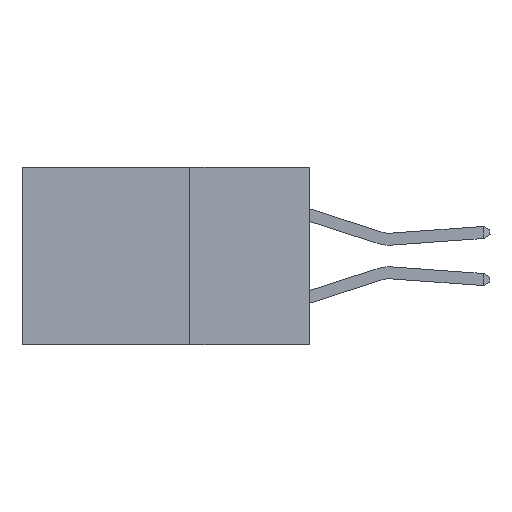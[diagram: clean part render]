
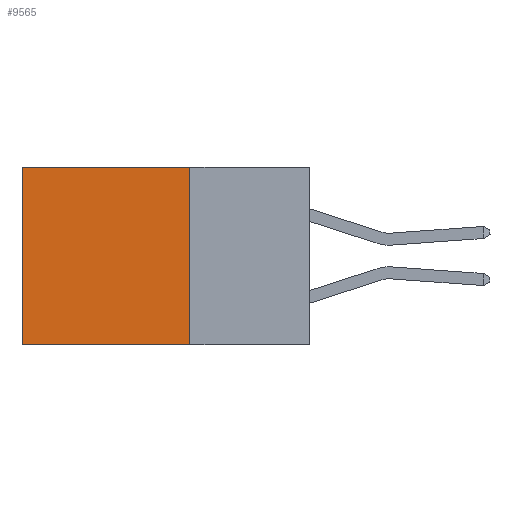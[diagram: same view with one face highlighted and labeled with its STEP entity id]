
A CAD part, left-side view. The second image highlights one B-rep face of the part: STEP entity #9565.
In plain terms, the highlighted planar face has unit normal (-1, 0, 0).
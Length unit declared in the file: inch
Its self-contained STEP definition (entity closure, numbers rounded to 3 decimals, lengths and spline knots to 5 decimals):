
#216 = CARTESIAN_POINT ( 'NONE',  ( 0.2615, 0.25, -0.37 ) ) ;
#240 = PLANE ( 'NONE',  #24524 ) ;
#1861 = CARTESIAN_POINT ( 'NONE',  ( 0.2615, 0.25, -0.37 ) ) ;
#1886 = DIRECTION ( 'NONE',  ( 0., 1., 0. ) ) ;
#2394 = DIRECTION ( 'NONE',  ( 1., 0., 0. ) ) ;
#2486 = VECTOR ( 'NONE', #1886, 39.37008 ) ;
#3098 = EDGE_CURVE ( 'NONE', #16211, #21364, #10154, .T. ) ;
#4338 = ORIENTED_EDGE ( 'NONE', *, *, #3098, .F. ) ;
#4615 = EDGE_CURVE ( 'NONE', #16211, #14962, #7761, .T. ) ;
#4818 = ORIENTED_EDGE ( 'NONE', *, *, #16704, .T. ) ;
#5083 = ORIENTED_EDGE ( 'NONE', *, *, #7350, .F. ) ;
#7350 = EDGE_CURVE ( 'NONE', #21364, #23464, #8261, .T. ) ;
#7761 = LINE ( 'NONE', #14718, #18285 ) ;
#8261 = LINE ( 'NONE', #1861, #2486 ) ;
#9317 = CARTESIAN_POINT ( 'NONE',  ( 0.2615, 0.25, -0.37 ) ) ;
#9565 = ADVANCED_FACE ( 'NONE', ( #9933 ), #240, .F. ) ;
#9933 = FACE_OUTER_BOUND ( 'NONE', #15324, .T. ) ;
#10154 = LINE ( 'NONE', #9317, #15082 ) ;
#10200 = ORIENTED_EDGE ( 'NONE', *, *, #4615, .T. ) ;
#12966 = CARTESIAN_POINT ( 'NONE',  ( 0.2615, 0.25, 0. ) ) ;
#13138 = CARTESIAN_POINT ( 'NONE',  ( 0.2615, 0.25, -0.37 ) ) ;
#14632 = VECTOR ( 'NONE', #23030, 39.37008 ) ;
#14712 = DIRECTION ( 'NONE',  ( 0., 1., 0. ) ) ;
#14718 = CARTESIAN_POINT ( 'NONE',  ( 0.2615, 0.25, 0. ) ) ;
#14773 = CARTESIAN_POINT ( 'NONE',  ( 0.2615, 0.6, -0.37 ) ) ;
#14962 = VERTEX_POINT ( 'NONE', #17572 ) ;
#15082 = VECTOR ( 'NONE', #15519, 39.37008 ) ;
#15324 = EDGE_LOOP ( 'NONE', ( #4818, #5083, #4338, #10200 ) ) ;
#15519 = DIRECTION ( 'NONE',  ( 0., 0., -1. ) ) ;
#16211 = VERTEX_POINT ( 'NONE', #12966 ) ;
#16704 = EDGE_CURVE ( 'NONE', #14962, #23464, #20141, .T. ) ;
#17303 = CARTESIAN_POINT ( 'NONE',  ( 0.2615, 0.6, -0.37 ) ) ;
#17319 = DIRECTION ( 'NONE',  ( 0., 0., -1. ) ) ;
#17572 = CARTESIAN_POINT ( 'NONE',  ( 0.2615, 0.6, 0. ) ) ;
#18285 = VECTOR ( 'NONE', #14712, 39.37008 ) ;
#20141 = LINE ( 'NONE', #14773, #14632 ) ;
#21364 = VERTEX_POINT ( 'NONE', #216 ) ;
#23030 = DIRECTION ( 'NONE',  ( 0., 0., -1. ) ) ;
#23464 = VERTEX_POINT ( 'NONE', #17303 ) ;
#24524 = AXIS2_PLACEMENT_3D ( 'NONE', #13138, #2394, #17319 ) ;
